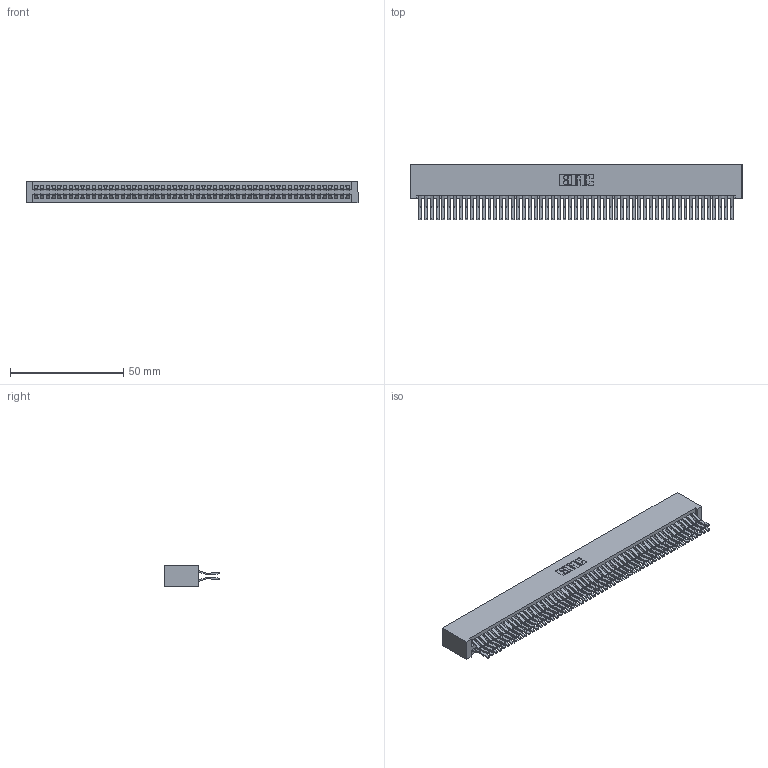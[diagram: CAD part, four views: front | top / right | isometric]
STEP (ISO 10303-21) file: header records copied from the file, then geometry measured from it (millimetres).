
FILE_DESCRIPTION (( 'STEP AP203' ), '1' );
FILE_NAME ('395-110-560-201.STEP', '2019-10-27T12:29:54', ( '' ), ( '' ), 'SwSTEP 2.0', 'SolidWorks 2016', '' );
FILE_SCHEMA (( 'CONFIG_CONTROL_DESIGN' ));
Length unit declared in the file: inch
Products named in the file (3): 345 Part_No Mounting Lugs; 345-292-001_560 Tail; 395-110-560-201
Assembly tree (111 placements, depth 2):
  395-110-560-201
    345 Part_No Mounting Lugs
    345-292-001_560 Tail  x110
Bounding box: 146.3 x 24.45 x 9.4 mm (x, y, z)
Volume: 15669.7 mm3; surface area: 25571.9 mm2
Topology: 111 solids, 111 shells, 5838 faces, 17367 edges, 11430 vertices
Faces by surface type: plane 3706, cylinder 2132
Entity records: 41215 total; most frequent: CARTESIAN_POINT 6896, ORIENTED_EDGE 6830, DIRECTION 6063, EDGE_CURVE 3415, LINE 3067, VECTOR 3067, VERTEX_POINT 2274, AXIS2_PLACEMENT_3D 1498
